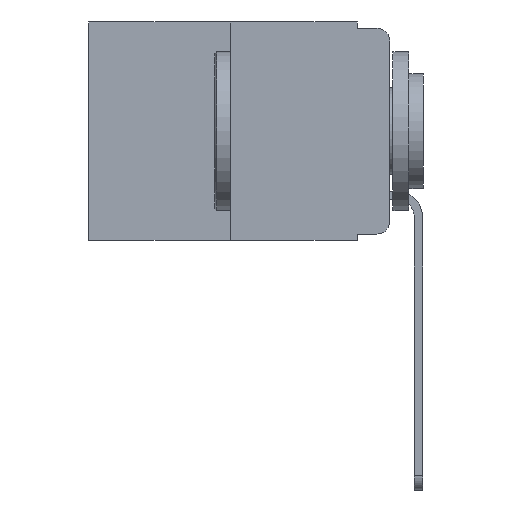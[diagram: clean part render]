
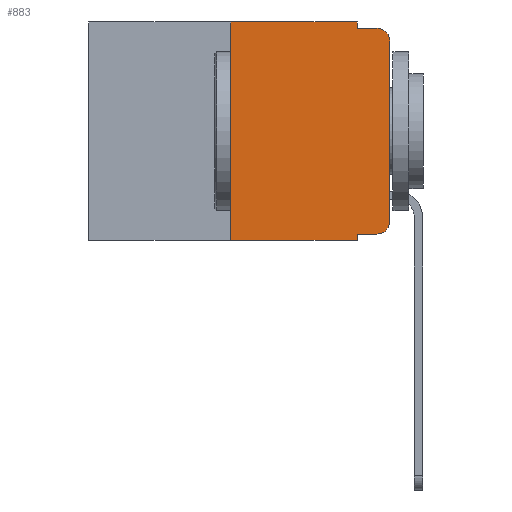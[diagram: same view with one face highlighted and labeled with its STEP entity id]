
A CAD part, left-side view. The second image highlights one B-rep face of the part: STEP entity #883.
In plain terms, the highlighted planar face has unit normal (-1, 0, 0).
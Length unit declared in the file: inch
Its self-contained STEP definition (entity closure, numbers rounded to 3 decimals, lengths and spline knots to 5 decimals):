
#113 = ORIENTED_EDGE ( 'NONE', *, *, #486, .T. ) ;
#401 = CIRCLE ( 'NONE', #4813, 0.02 ) ;
#486 = EDGE_CURVE ( 'NONE', #13032, #11639, #6775, .T. ) ;
#750 = ORIENTED_EDGE ( 'NONE', *, *, #12438, .F. ) ;
#805 = CARTESIAN_POINT ( 'NONE',  ( 0., 0.051, 0. ) ) ;
#883 = ADVANCED_FACE ( 'NONE', ( #7414 ), #9985, .F. ) ;
#1148 = ORIENTED_EDGE ( 'NONE', *, *, #8181, .T. ) ;
#1394 = VERTEX_POINT ( 'NONE', #11794 ) ;
#1448 = ORIENTED_EDGE ( 'NONE', *, *, #4823, .F. ) ;
#1804 = CARTESIAN_POINT ( 'NONE',  ( 0., 0.051, 0. ) ) ;
#1938 = CARTESIAN_POINT ( 'NONE',  ( 0., 0.051, -0.343 ) ) ;
#2306 = VERTEX_POINT ( 'NONE', #6512 ) ;
#2389 = LINE ( 'NONE', #6414, #7567 ) ;
#2457 = CARTESIAN_POINT ( 'NONE',  ( 0., 0.051, -0.01 ) ) ;
#2541 = VECTOR ( 'NONE', #6127, 39.37008 ) ;
#2572 = VERTEX_POINT ( 'NONE', #8063 ) ;
#2657 = CIRCLE ( 'NONE', #8141, 0.02 ) ;
#2684 = LINE ( 'NONE', #9226, #6073 ) ;
#2848 = EDGE_CURVE ( 'NONE', #4860, #12853, #2389, .T. ) ;
#3015 = VERTEX_POINT ( 'NONE', #3730 ) ;
#3461 = LINE ( 'NONE', #805, #3782 ) ;
#3647 = VECTOR ( 'NONE', #5563, 39.37008 ) ;
#3671 = LINE ( 'NONE', #8667, #11607 ) ;
#3730 = CARTESIAN_POINT ( 'NONE',  ( 0., 0., -0.313 ) ) ;
#3782 = VECTOR ( 'NONE', #8060, 39.37008 ) ;
#3958 = EDGE_CURVE ( 'NONE', #12853, #3015, #401, .T. ) ;
#4154 = CARTESIAN_POINT ( 'NONE',  ( 0., 0.25, 0. ) ) ;
#4727 = CARTESIAN_POINT ( 'NONE',  ( 0., 0.02, -0.03 ) ) ;
#4795 = DIRECTION ( 'NONE',  ( 0., 0., -1. ) ) ;
#4813 = AXIS2_PLACEMENT_3D ( 'NONE', #11491, #5278, #12518 ) ;
#4823 = EDGE_CURVE ( 'NONE', #1394, #2572, #6385, .T. ) ;
#4860 = VERTEX_POINT ( 'NONE', #11859 ) ;
#5042 = VERTEX_POINT ( 'NONE', #1804 ) ;
#5278 = DIRECTION ( 'NONE',  ( -1., 0., 0. ) ) ;
#5524 = EDGE_CURVE ( 'NONE', #4860, #11639, #3461, .T. ) ;
#5563 = DIRECTION ( 'NONE',  ( 0., -1., 0. ) ) ;
#5769 = DIRECTION ( 'NONE',  ( 0., 0., -1. ) ) ;
#6011 = EDGE_LOOP ( 'NONE', ( #9099, #1148, #1448, #7758, #750, #6088, #113, #10096, #6525, #8603 ) ) ;
#6073 = VECTOR ( 'NONE', #13357, 39.37008 ) ;
#6088 = ORIENTED_EDGE ( 'NONE', *, *, #6703, .F. ) ;
#6127 = DIRECTION ( 'NONE',  ( 0., 0., 1. ) ) ;
#6215 = CARTESIAN_POINT ( 'NONE',  ( 0., 0.02, -0.333 ) ) ;
#6293 = DIRECTION ( 'NONE',  ( 0., -1., 0. ) ) ;
#6385 = LINE ( 'NONE', #2457, #3647 ) ;
#6414 = CARTESIAN_POINT ( 'NONE',  ( 0., 0.051, -0.333 ) ) ;
#6482 = CARTESIAN_POINT ( 'NONE',  ( 0., 0.25, -0.343 ) ) ;
#6512 = CARTESIAN_POINT ( 'NONE',  ( 0., 0., -0.03 ) ) ;
#6525 = ORIENTED_EDGE ( 'NONE', *, *, #2848, .T. ) ;
#6545 = EDGE_CURVE ( 'NONE', #3015, #2306, #8047, .T. ) ;
#6703 = EDGE_CURVE ( 'NONE', #13032, #10424, #3671, .T. ) ;
#6775 = LINE ( 'NONE', #9407, #9223 ) ;
#7142 = VECTOR ( 'NONE', #12700, 39.37008 ) ;
#7414 = FACE_OUTER_BOUND ( 'NONE', #6011, .T. ) ;
#7567 = VECTOR ( 'NONE', #10596, 39.37008 ) ;
#7758 = ORIENTED_EDGE ( 'NONE', *, *, #9086, .F. ) ;
#8047 = LINE ( 'NONE', #8162, #2541 ) ;
#8060 = DIRECTION ( 'NONE',  ( 0., 0., -1. ) ) ;
#8063 = CARTESIAN_POINT ( 'NONE',  ( 0., 0.02, -0.01 ) ) ;
#8141 = AXIS2_PLACEMENT_3D ( 'NONE', #4727, #11971, #5769 ) ;
#8162 = CARTESIAN_POINT ( 'NONE',  ( 0., 0., 0. ) ) ;
#8181 = EDGE_CURVE ( 'NONE', #2306, #2572, #2657, .T. ) ;
#8184 = AXIS2_PLACEMENT_3D ( 'NONE', #13028, #11011, #4795 ) ;
#8603 = ORIENTED_EDGE ( 'NONE', *, *, #3958, .T. ) ;
#8667 = CARTESIAN_POINT ( 'NONE',  ( 0., 0.25, 0. ) ) ;
#9086 = EDGE_CURVE ( 'NONE', #5042, #1394, #2684, .T. ) ;
#9099 = ORIENTED_EDGE ( 'NONE', *, *, #6545, .T. ) ;
#9223 = VECTOR ( 'NONE', #6293, 39.37008 ) ;
#9226 = CARTESIAN_POINT ( 'NONE',  ( 0., 0.051, 0. ) ) ;
#9407 = CARTESIAN_POINT ( 'NONE',  ( 0., 0.473, -0.343 ) ) ;
#9655 = CARTESIAN_POINT ( 'NONE',  ( 0., 0.473, 0. ) ) ;
#9985 = PLANE ( 'NONE',  #8184 ) ;
#10096 = ORIENTED_EDGE ( 'NONE', *, *, #5524, .F. ) ;
#10424 = VERTEX_POINT ( 'NONE', #4154 ) ;
#10596 = DIRECTION ( 'NONE',  ( 0., -1., 0. ) ) ;
#11011 = DIRECTION ( 'NONE',  ( 1., 0., 0. ) ) ;
#11491 = CARTESIAN_POINT ( 'NONE',  ( 0., 0.02, -0.313 ) ) ;
#11607 = VECTOR ( 'NONE', #12771, 39.37008 ) ;
#11639 = VERTEX_POINT ( 'NONE', #1938 ) ;
#11794 = CARTESIAN_POINT ( 'NONE',  ( 0., 0.051, -0.01 ) ) ;
#11859 = CARTESIAN_POINT ( 'NONE',  ( 0., 0.051, -0.333 ) ) ;
#11971 = DIRECTION ( 'NONE',  ( -1., 0., 0. ) ) ;
#12438 = EDGE_CURVE ( 'NONE', #10424, #5042, #12649, .T. ) ;
#12518 = DIRECTION ( 'NONE',  ( 0., 0., -1. ) ) ;
#12649 = LINE ( 'NONE', #9655, #7142 ) ;
#12700 = DIRECTION ( 'NONE',  ( 0., -1., 0. ) ) ;
#12771 = DIRECTION ( 'NONE',  ( 0., 0., 1. ) ) ;
#12853 = VERTEX_POINT ( 'NONE', #6215 ) ;
#13028 = CARTESIAN_POINT ( 'NONE',  ( 0., 0.473, 0. ) ) ;
#13032 = VERTEX_POINT ( 'NONE', #6482 ) ;
#13357 = DIRECTION ( 'NONE',  ( 0., 0., -1. ) ) ;
